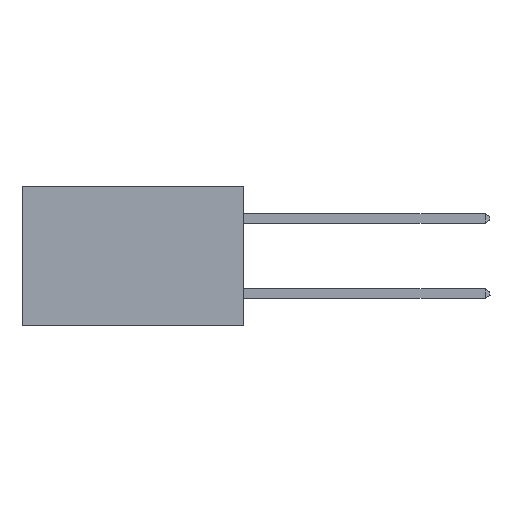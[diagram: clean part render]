
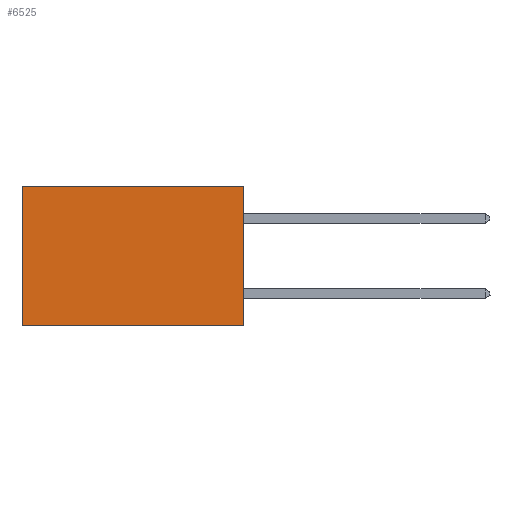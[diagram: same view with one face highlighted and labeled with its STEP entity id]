
A CAD part, left-side view. The second image highlights one B-rep face of the part: STEP entity #6525.
In plain terms, the highlighted planar face has unit normal (-1, 0, 0).
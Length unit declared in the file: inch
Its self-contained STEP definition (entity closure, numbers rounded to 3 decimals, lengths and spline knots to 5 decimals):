
#359 = VERTEX_POINT ( 'NONE', #12107 ) ;
#872 = DIRECTION ( 'NONE',  ( 1., 0., 0. ) ) ;
#1885 = CARTESIAN_POINT ( 'NONE',  ( 0.277, 0.59, -0.37 ) ) ;
#2489 = DIRECTION ( 'NONE',  ( 0., 0., -1. ) ) ;
#3079 = DIRECTION ( 'NONE',  ( 0., 0., -1. ) ) ;
#3259 = EDGE_CURVE ( 'NONE', #359, #10117, #14970, .T. ) ;
#4026 = EDGE_LOOP ( 'NONE', ( #7552, #4097, #4621, #14663 ) ) ;
#4097 = ORIENTED_EDGE ( 'NONE', *, *, #14137, .F. ) ;
#4368 = DIRECTION ( 'NONE',  ( 0., 1., 0. ) ) ;
#4621 = ORIENTED_EDGE ( 'NONE', *, *, #5757, .F. ) ;
#4683 = VECTOR ( 'NONE', #3079, 39.37008 ) ;
#5508 = CARTESIAN_POINT ( 'NONE',  ( 0.277, 0., -0.37 ) ) ;
#5710 = CARTESIAN_POINT ( 'NONE',  ( 0.277, 0.59, -0.37 ) ) ;
#5757 = EDGE_CURVE ( 'NONE', #359, #9651, #5940, .T. ) ;
#5878 = VERTEX_POINT ( 'NONE', #5710 ) ;
#5940 = LINE ( 'NONE', #7172, #11866 ) ;
#6525 = ADVANCED_FACE ( 'NONE', ( #13712 ), #14027, .F. ) ;
#6530 = DIRECTION ( 'NONE',  ( 0., 1., 0. ) ) ;
#7141 = DIRECTION ( 'NONE',  ( 0., 0., -1. ) ) ;
#7168 = CARTESIAN_POINT ( 'NONE',  ( 0.277, 0., -0.37 ) ) ;
#7172 = CARTESIAN_POINT ( 'NONE',  ( 0.277, 0., -0.37 ) ) ;
#7552 = ORIENTED_EDGE ( 'NONE', *, *, #13243, .T. ) ;
#8207 = LINE ( 'NONE', #1885, #4683 ) ;
#8349 = VECTOR ( 'NONE', #4368, 39.37008 ) ;
#8846 = CARTESIAN_POINT ( 'NONE',  ( 0.277, 0., -0.37 ) ) ;
#9651 = VERTEX_POINT ( 'NONE', #5508 ) ;
#9846 = CARTESIAN_POINT ( 'NONE',  ( 0.277, 0.59, 0. ) ) ;
#10117 = VERTEX_POINT ( 'NONE', #9846 ) ;
#11866 = VECTOR ( 'NONE', #7141, 39.37008 ) ;
#12107 = CARTESIAN_POINT ( 'NONE',  ( 0.277, 0., 0. ) ) ;
#13243 = EDGE_CURVE ( 'NONE', #10117, #5878, #8207, .T. ) ;
#13327 = AXIS2_PLACEMENT_3D ( 'NONE', #7168, #872, #2489 ) ;
#13371 = VECTOR ( 'NONE', #6530, 39.37008 ) ;
#13712 = FACE_OUTER_BOUND ( 'NONE', #4026, .T. ) ;
#13740 = LINE ( 'NONE', #8846, #13371 ) ;
#14027 = PLANE ( 'NONE',  #13327 ) ;
#14137 = EDGE_CURVE ( 'NONE', #9651, #5878, #13740, .T. ) ;
#14663 = ORIENTED_EDGE ( 'NONE', *, *, #3259, .T. ) ;
#14970 = LINE ( 'NONE', #15066, #8349 ) ;
#15066 = CARTESIAN_POINT ( 'NONE',  ( 0.277, 0., 0. ) ) ;
